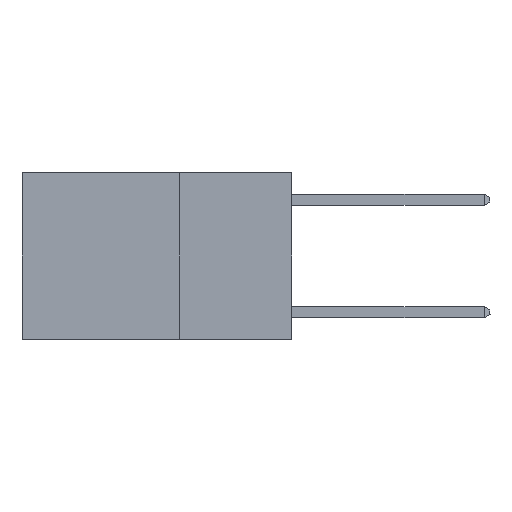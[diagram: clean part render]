
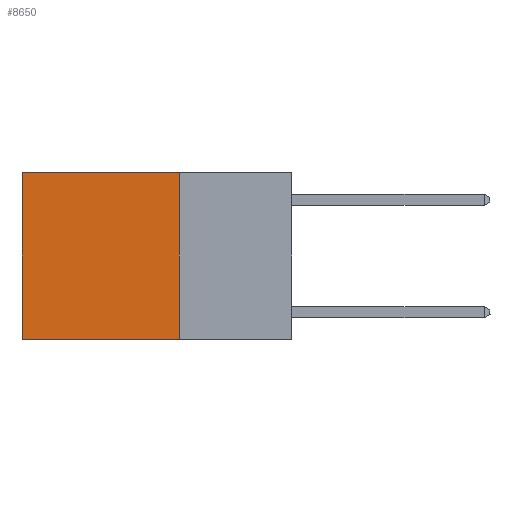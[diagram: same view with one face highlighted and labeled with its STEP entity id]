
A CAD part, left-side view. The second image highlights one B-rep face of the part: STEP entity #8650.
In plain terms, the highlighted planar face has unit normal (-1, 0, 0).
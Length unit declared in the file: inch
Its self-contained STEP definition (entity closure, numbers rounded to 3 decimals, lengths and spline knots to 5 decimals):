
#1700 = VERTEX_POINT ( 'NONE', #3986 ) ;
#1896 = DIRECTION ( 'NONE',  ( 0., 1., 0. ) ) ;
#1910 = LINE ( 'NONE', #20835, #7198 ) ;
#2498 = DIRECTION ( 'NONE',  ( 0., 1., 0. ) ) ;
#3716 = VECTOR ( 'NONE', #2498, 39.37008 ) ;
#3986 = CARTESIAN_POINT ( 'NONE',  ( 0.2625, 0.6, 0. ) ) ;
#4115 = AXIS2_PLACEMENT_3D ( 'NONE', #6320, #18438, #8213 ) ;
#4348 = PLANE ( 'NONE',  #4115 ) ;
#5272 = CARTESIAN_POINT ( 'NONE',  ( 0.2625, 0.25, -0.37 ) ) ;
#5726 = EDGE_CURVE ( 'NONE', #20554, #7862, #1910, .T. ) ;
#6320 = CARTESIAN_POINT ( 'NONE',  ( 0.2625, 0.25, 0. ) ) ;
#7198 = VECTOR ( 'NONE', #19193, 39.37008 ) ;
#7862 = VERTEX_POINT ( 'NONE', #5272 ) ;
#8213 = DIRECTION ( 'NONE',  ( 0., 0., -1. ) ) ;
#8478 = VERTEX_POINT ( 'NONE', #12774 ) ;
#8650 = ADVANCED_FACE ( 'NONE', ( #9047 ), #4348, .F. ) ;
#9047 = FACE_OUTER_BOUND ( 'NONE', #11531, .T. ) ;
#9384 = LINE ( 'NONE', #20138, #3716 ) ;
#10410 = EDGE_CURVE ( 'NONE', #1700, #8478, #17809, .T. ) ;
#11123 = EDGE_CURVE ( 'NONE', #20554, #1700, #13596, .T. ) ;
#11531 = EDGE_LOOP ( 'NONE', ( #11949, #12047, #12134, #12309 ) ) ;
#11949 = ORIENTED_EDGE ( 'NONE', *, *, #10410, .T. ) ;
#12047 = ORIENTED_EDGE ( 'NONE', *, *, #14591, .F. ) ;
#12134 = ORIENTED_EDGE ( 'NONE', *, *, #5726, .F. ) ;
#12309 = ORIENTED_EDGE ( 'NONE', *, *, #11123, .T. ) ;
#12774 = CARTESIAN_POINT ( 'NONE',  ( 0.2625, 0.6, -0.37 ) ) ;
#13179 = CARTESIAN_POINT ( 'NONE',  ( 0.2625, 0.6, 0. ) ) ;
#13346 = VECTOR ( 'NONE', #19739, 39.37008 ) ;
#13596 = LINE ( 'NONE', #21316, #17513 ) ;
#14591 = EDGE_CURVE ( 'NONE', #7862, #8478, #9384, .T. ) ;
#17513 = VECTOR ( 'NONE', #1896, 39.37008 ) ;
#17809 = LINE ( 'NONE', #13179, #13346 ) ;
#18242 = CARTESIAN_POINT ( 'NONE',  ( 0.2625, 0.25, 0. ) ) ;
#18438 = DIRECTION ( 'NONE',  ( 1., 0., 0. ) ) ;
#19193 = DIRECTION ( 'NONE',  ( 0., 0., -1. ) ) ;
#19739 = DIRECTION ( 'NONE',  ( 0., 0., -1. ) ) ;
#20138 = CARTESIAN_POINT ( 'NONE',  ( 0.2625, 0.25, -0.37 ) ) ;
#20554 = VERTEX_POINT ( 'NONE', #18242 ) ;
#20835 = CARTESIAN_POINT ( 'NONE',  ( 0.2625, 0.25, 0. ) ) ;
#21316 = CARTESIAN_POINT ( 'NONE',  ( 0.2625, 0.25, 0. ) ) ;
